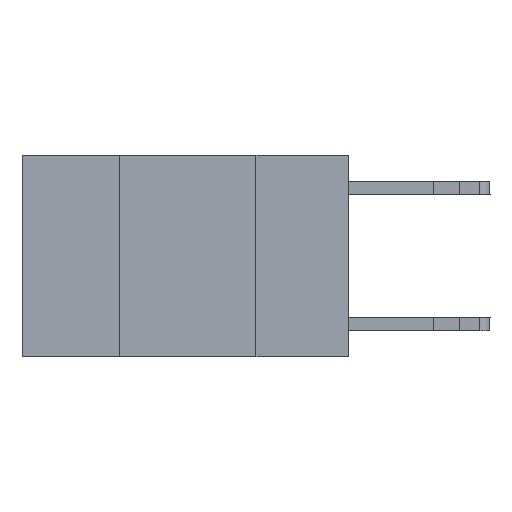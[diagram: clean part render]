
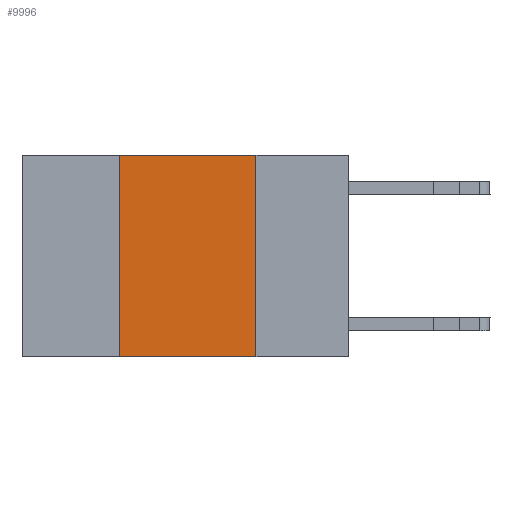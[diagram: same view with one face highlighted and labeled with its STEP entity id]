
A CAD part, left-side view. The second image highlights one B-rep face of the part: STEP entity #9996.
In plain terms, the highlighted planar face has unit normal (-1, 0, 0).
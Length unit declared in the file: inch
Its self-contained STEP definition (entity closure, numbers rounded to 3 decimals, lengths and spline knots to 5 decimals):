
#270 = CARTESIAN_POINT ( 'NONE',  ( 0., 0.6, 0. ) ) ;
#524 = AXIS2_PLACEMENT_3D ( 'NONE', #270, #5537, #6981 ) ;
#552 = CARTESIAN_POINT ( 'NONE',  ( 0., 0.42, 0. ) ) ;
#1529 = FACE_OUTER_BOUND ( 'NONE', #4463, .T. ) ;
#1685 = VERTEX_POINT ( 'NONE', #13784 ) ;
#2118 = EDGE_CURVE ( 'NONE', #2955, #16746, #7103, .T. ) ;
#2246 = LINE ( 'NONE', #10104, #7391 ) ;
#2955 = VERTEX_POINT ( 'NONE', #3006 ) ;
#3006 = CARTESIAN_POINT ( 'NONE',  ( 0., 0.42, -0.37 ) ) ;
#3715 = LINE ( 'NONE', #14433, #13452 ) ;
#3937 = CARTESIAN_POINT ( 'NONE',  ( 0., 0.17, 0. ) ) ;
#4206 = EDGE_CURVE ( 'NONE', #16746, #14308, #2246, .T. ) ;
#4463 = EDGE_LOOP ( 'NONE', ( #10548, #14663, #11873, #13328 ) ) ;
#4549 = VECTOR ( 'NONE', #5350, 39.37008 ) ;
#5350 = DIRECTION ( 'NONE',  ( 0., 0., 1. ) ) ;
#5537 = DIRECTION ( 'NONE',  ( 1., 0., 0. ) ) ;
#5970 = CARTESIAN_POINT ( 'NONE',  ( 0., 0.42, 0. ) ) ;
#6981 = DIRECTION ( 'NONE',  ( 0., 0., -1. ) ) ;
#7103 = LINE ( 'NONE', #552, #4549 ) ;
#7391 = VECTOR ( 'NONE', #8812, 39.37008 ) ;
#7826 = LINE ( 'NONE', #3937, #9169 ) ;
#8812 = DIRECTION ( 'NONE',  ( 0., -1., 0. ) ) ;
#9169 = VECTOR ( 'NONE', #9189, 39.37008 ) ;
#9189 = DIRECTION ( 'NONE',  ( 0., 0., -1. ) ) ;
#9752 = EDGE_CURVE ( 'NONE', #2955, #1685, #3715, .T. ) ;
#9996 = ADVANCED_FACE ( 'NONE', ( #1529 ), #10865, .F. ) ;
#10104 = CARTESIAN_POINT ( 'NONE',  ( 0., 0.6, 0. ) ) ;
#10548 = ORIENTED_EDGE ( 'NONE', *, *, #10971, .F. ) ;
#10865 = PLANE ( 'NONE',  #524 ) ;
#10971 = EDGE_CURVE ( 'NONE', #14308, #1685, #7826, .T. ) ;
#11873 = ORIENTED_EDGE ( 'NONE', *, *, #2118, .F. ) ;
#13328 = ORIENTED_EDGE ( 'NONE', *, *, #9752, .T. ) ;
#13452 = VECTOR ( 'NONE', #16845, 39.37008 ) ;
#13784 = CARTESIAN_POINT ( 'NONE',  ( 0., 0.17, -0.37 ) ) ;
#14308 = VERTEX_POINT ( 'NONE', #16437 ) ;
#14433 = CARTESIAN_POINT ( 'NONE',  ( 0., 0.6, -0.37 ) ) ;
#14663 = ORIENTED_EDGE ( 'NONE', *, *, #4206, .F. ) ;
#16437 = CARTESIAN_POINT ( 'NONE',  ( 0., 0.17, 0. ) ) ;
#16746 = VERTEX_POINT ( 'NONE', #5970 ) ;
#16845 = DIRECTION ( 'NONE',  ( 0., -1., 0. ) ) ;
